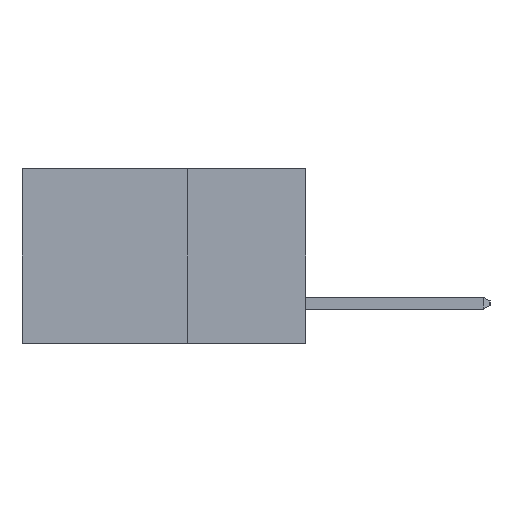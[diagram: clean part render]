
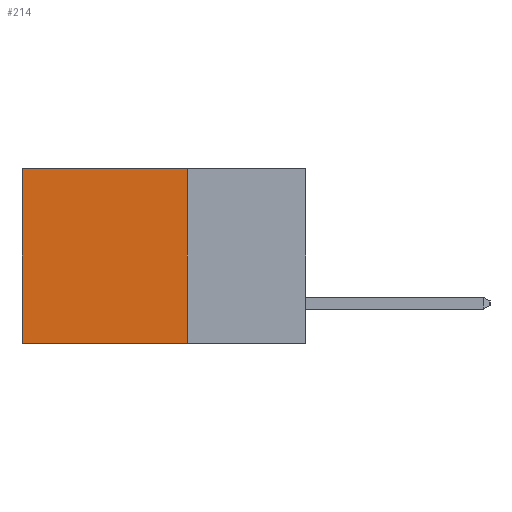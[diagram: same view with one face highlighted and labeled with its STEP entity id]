
A CAD part, left-side view. The second image highlights one B-rep face of the part: STEP entity #214.
In plain terms, the highlighted planar face has unit normal (-1, 0, 0).
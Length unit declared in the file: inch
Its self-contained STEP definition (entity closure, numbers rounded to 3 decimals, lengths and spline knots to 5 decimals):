
#214 = ADVANCED_FACE ( 'NONE', ( #15696 ), #2628, .F. ) ;
#289 = LINE ( 'NONE', #14412, #10982 ) ;
#639 = LINE ( 'NONE', #14676, #3545 ) ;
#1034 = AXIS2_PLACEMENT_3D ( 'NONE', #5324, #13650, #13629 ) ;
#1090 = LINE ( 'NONE', #2243, #8139 ) ;
#2159 = CARTESIAN_POINT ( 'NONE',  ( 0.298, 0.6, 0. ) ) ;
#2235 = EDGE_CURVE ( 'NONE', #5354, #5083, #289, .T. ) ;
#2243 = CARTESIAN_POINT ( 'NONE',  ( 0.298, 0.25, 0. ) ) ;
#2628 = PLANE ( 'NONE',  #1034 ) ;
#3545 = VECTOR ( 'NONE', #5183, 39.37008 ) ;
#3667 = DIRECTION ( 'NONE',  ( 0., 1., 0. ) ) ;
#3858 = EDGE_LOOP ( 'NONE', ( #3920, #6787, #8233, #4929 ) ) ;
#3920 = ORIENTED_EDGE ( 'NONE', *, *, #2235, .T. ) ;
#4929 = ORIENTED_EDGE ( 'NONE', *, *, #12002, .T. ) ;
#5083 = VERTEX_POINT ( 'NONE', #16502 ) ;
#5183 = DIRECTION ( 'NONE',  ( 0., 1., 0. ) ) ;
#5324 = CARTESIAN_POINT ( 'NONE',  ( 0.298, 0.25, 0. ) ) ;
#5354 = VERTEX_POINT ( 'NONE', #2159 ) ;
#5448 = EDGE_CURVE ( 'NONE', #7890, #5083, #639, .T. ) ;
#6787 = ORIENTED_EDGE ( 'NONE', *, *, #5448, .F. ) ;
#7481 = LINE ( 'NONE', #11105, #13785 ) ;
#7890 = VERTEX_POINT ( 'NONE', #17047 ) ;
#8139 = VECTOR ( 'NONE', #3667, 39.37008 ) ;
#8233 = ORIENTED_EDGE ( 'NONE', *, *, #12254, .F. ) ;
#10150 = CARTESIAN_POINT ( 'NONE',  ( 0.298, 0.25, 0. ) ) ;
#10892 = DIRECTION ( 'NONE',  ( 0., 0., -1. ) ) ;
#10982 = VECTOR ( 'NONE', #10892, 39.37008 ) ;
#11105 = CARTESIAN_POINT ( 'NONE',  ( 0.298, 0.25, 0. ) ) ;
#12002 = EDGE_CURVE ( 'NONE', #15124, #5354, #1090, .T. ) ;
#12254 = EDGE_CURVE ( 'NONE', #15124, #7890, #7481, .T. ) ;
#12453 = DIRECTION ( 'NONE',  ( 0., 0., -1. ) ) ;
#13629 = DIRECTION ( 'NONE',  ( 0., 0., -1. ) ) ;
#13650 = DIRECTION ( 'NONE',  ( 1., 0., 0. ) ) ;
#13785 = VECTOR ( 'NONE', #12453, 39.37008 ) ;
#14412 = CARTESIAN_POINT ( 'NONE',  ( 0.298, 0.6, 0. ) ) ;
#14676 = CARTESIAN_POINT ( 'NONE',  ( 0.298, 0.25, -0.37 ) ) ;
#15124 = VERTEX_POINT ( 'NONE', #10150 ) ;
#15696 = FACE_OUTER_BOUND ( 'NONE', #3858, .T. ) ;
#16502 = CARTESIAN_POINT ( 'NONE',  ( 0.298, 0.6, -0.37 ) ) ;
#17047 = CARTESIAN_POINT ( 'NONE',  ( 0.298, 0.25, -0.37 ) ) ;
